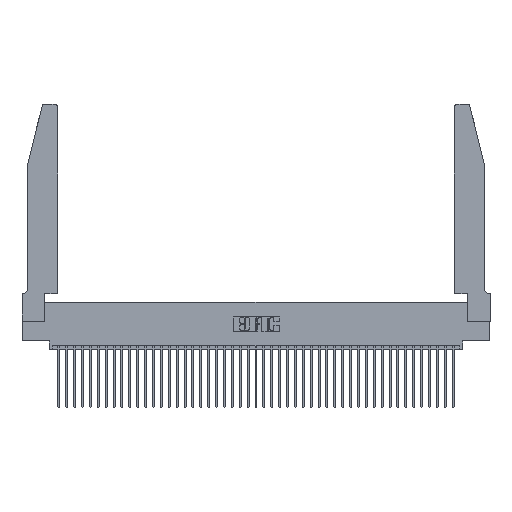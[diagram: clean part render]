
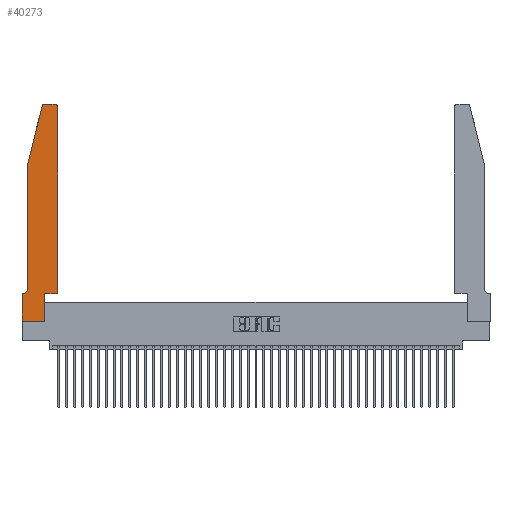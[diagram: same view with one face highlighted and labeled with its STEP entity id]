
A CAD part, top view. The second image highlights one B-rep face of the part: STEP entity #40273.
In plain terms, the highlighted planar face has unit normal (0, 0, 1).
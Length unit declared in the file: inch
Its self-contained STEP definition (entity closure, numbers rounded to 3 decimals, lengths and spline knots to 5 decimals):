
#935 = DIRECTION ( 'NONE',  ( -1., 0., 0. ) ) ;
#1288 = DIRECTION ( 'NONE',  ( 1., 0., 0. ) ) ;
#3307 = DIRECTION ( 'NONE',  ( 0., -1., 0. ) ) ;
#3815 = VERTEX_POINT ( 'NONE', #11834 ) ;
#4508 = CARTESIAN_POINT ( 'NONE',  ( 0.2865, 0., 0.37 ) ) ;
#4598 = EDGE_LOOP ( 'NONE', ( #22814, #32112, #6615, #11169, #37829, #42967, #33319, #41720, #20556, #8556, #37438, #32371 ) ) ;
#5459 = VECTOR ( 'NONE', #7667, 39.37008 ) ;
#5753 = DIRECTION ( 'NONE',  ( 1., 0., 0. ) ) ;
#6615 = ORIENTED_EDGE ( 'NONE', *, *, #26195, .T. ) ;
#6914 = DIRECTION ( 'NONE',  ( 1., 0., 0. ) ) ;
#7610 = CARTESIAN_POINT ( 'NONE',  ( 0.0755, 2., 0.37 ) ) ;
#7634 = CARTESIAN_POINT ( 'NONE',  ( 0., 0., 0.37 ) ) ;
#7667 = DIRECTION ( 'NONE',  ( -1., 0., 0. ) ) ;
#8154 = EDGE_CURVE ( 'NONE', #12439, #22724, #13088, .T. ) ;
#8410 = VERTEX_POINT ( 'NONE', #4508 ) ;
#8518 = CARTESIAN_POINT ( 'NONE',  ( 0.2865, 0.35, 0.37 ) ) ;
#8556 = ORIENTED_EDGE ( 'NONE', *, *, #33210, .T. ) ;
#9580 = CARTESIAN_POINT ( 'NONE',  ( 0.4205, 2.75, 0.37 ) ) ;
#9873 = CARTESIAN_POINT ( 'NONE',  ( 0.25487, 2.72718, 0.37 ) ) ;
#10303 = CARTESIAN_POINT ( 'NONE',  ( 0.2605, 2.75, 0.37 ) ) ;
#10686 = VECTOR ( 'NONE', #33899, 39.37008 ) ;
#11095 = EDGE_CURVE ( 'NONE', #3815, #42620, #15480, .T. ) ;
#11169 = ORIENTED_EDGE ( 'NONE', *, *, #31546, .T. ) ;
#11187 = DIRECTION ( 'NONE',  ( -0.239, -0.971, 0. ) ) ;
#11375 = DIRECTION ( 'NONE',  ( 0., 1., 0. ) ) ;
#11556 = VERTEX_POINT ( 'NONE', #36899 ) ;
#11834 = CARTESIAN_POINT ( 'NONE',  ( 0., 0.35, 0.37 ) ) ;
#12362 = VERTEX_POINT ( 'NONE', #9580 ) ;
#12417 = CARTESIAN_POINT ( 'NONE',  ( 0.4505, 0.35, 0.37 ) ) ;
#12439 = VERTEX_POINT ( 'NONE', #29566 ) ;
#12839 = LINE ( 'NONE', #12417, #37230 ) ;
#13063 = AXIS2_PLACEMENT_3D ( 'NONE', #14311, #21127, #935 ) ;
#13088 = CIRCLE ( 'NONE', #13063, 0.07 ) ;
#13174 = AXIS2_PLACEMENT_3D ( 'NONE', #28355, #38923, #1288 ) ;
#13742 = LINE ( 'NONE', #7610, #37541 ) ;
#14163 = CARTESIAN_POINT ( 'NONE',  ( 0.284, 2.72, 0.37 ) ) ;
#14311 = CARTESIAN_POINT ( 'NONE',  ( 0.0055, 0.42, 0.37 ) ) ;
#14461 = LINE ( 'NONE', #26041, #5459 ) ;
#15480 = LINE ( 'NONE', #23377, #32351 ) ;
#16044 = VERTEX_POINT ( 'NONE', #9873 ) ;
#16285 = DIRECTION ( 'NONE',  ( 0., -1., 0. ) ) ;
#16552 = CARTESIAN_POINT ( 'NONE',  ( 0.0055, 0.35, 0.37 ) ) ;
#16766 = CARTESIAN_POINT ( 'NONE',  ( 0.0755, 2., 0.37 ) ) ;
#17134 = CARTESIAN_POINT ( 'NONE',  ( 0.4205, 2.72, 0.37 ) ) ;
#18446 = VERTEX_POINT ( 'NONE', #36794 ) ;
#18506 = EDGE_CURVE ( 'NONE', #11556, #12362, #42036, .T. ) ;
#18605 = CARTESIAN_POINT ( 'NONE',  ( 0.2865, 0.35, 0.37 ) ) ;
#18828 = VECTOR ( 'NONE', #21265, 39.37008 ) ;
#20556 = ORIENTED_EDGE ( 'NONE', *, *, #22803, .T. ) ;
#21127 = DIRECTION ( 'NONE',  ( 0., 0., -1. ) ) ;
#21265 = DIRECTION ( 'NONE',  ( 0., 1., 0. ) ) ;
#21495 = PLANE ( 'NONE',  #13174 ) ;
#22724 = VERTEX_POINT ( 'NONE', #16552 ) ;
#22786 = VERTEX_POINT ( 'NONE', #30596 ) ;
#22803 = EDGE_CURVE ( 'NONE', #8410, #24852, #27697, .T. ) ;
#22814 = ORIENTED_EDGE ( 'NONE', *, *, #32704, .T. ) ;
#22847 = VERTEX_POINT ( 'NONE', #28722 ) ;
#23377 = CARTESIAN_POINT ( 'NONE',  ( 0., 0., 0.37 ) ) ;
#23465 = LINE ( 'NONE', #7634, #33442 ) ;
#24453 = FACE_OUTER_BOUND ( 'NONE', #4598, .T. ) ;
#24516 = DIRECTION ( 'NONE',  ( 0., 0., 1. ) ) ;
#24852 = VERTEX_POINT ( 'NONE', #8518 ) ;
#25799 = LINE ( 'NONE', #10303, #10686 ) ;
#26041 = CARTESIAN_POINT ( 'NONE',  ( 0.0755, 0.35, 0.37 ) ) ;
#26195 = EDGE_CURVE ( 'NONE', #16044, #18446, #13742, .T. ) ;
#27302 = EDGE_CURVE ( 'NONE', #22786, #11556, #34080, .T. ) ;
#27320 = EDGE_CURVE ( 'NONE', #22847, #16044, #33566, .T. ) ;
#27697 = LINE ( 'NONE', #18605, #43117 ) ;
#28355 = CARTESIAN_POINT ( 'NONE',  ( 0., 0.35, 0.37 ) ) ;
#28458 = CARTESIAN_POINT ( 'NONE',  ( 0., 0., 0.37 ) ) ;
#28722 = CARTESIAN_POINT ( 'NONE',  ( 0.284, 2.75, 0.37 ) ) ;
#29072 = AXIS2_PLACEMENT_3D ( 'NONE', #17134, #33640, #6914 ) ;
#29566 = CARTESIAN_POINT ( 'NONE',  ( 0.0755, 0.42, 0.37 ) ) ;
#30596 = CARTESIAN_POINT ( 'NONE',  ( 0.4505, 0.35, 0.37 ) ) ;
#31546 = EDGE_CURVE ( 'NONE', #18446, #12439, #41779, .T. ) ;
#31552 = CARTESIAN_POINT ( 'NONE',  ( 0.4505, 0.35, 0.37 ) ) ;
#32112 = ORIENTED_EDGE ( 'NONE', *, *, #27320, .T. ) ;
#32351 = VECTOR ( 'NONE', #16285, 39.37008 ) ;
#32371 = ORIENTED_EDGE ( 'NONE', *, *, #18506, .T. ) ;
#32704 = EDGE_CURVE ( 'NONE', #12362, #22847, #25799, .T. ) ;
#32716 = VECTOR ( 'NONE', #3307, 39.37008 ) ;
#32971 = AXIS2_PLACEMENT_3D ( 'NONE', #14163, #24516, #38118 ) ;
#33073 = EDGE_CURVE ( 'NONE', #22724, #3815, #14461, .T. ) ;
#33210 = EDGE_CURVE ( 'NONE', #24852, #22786, #12839, .T. ) ;
#33319 = ORIENTED_EDGE ( 'NONE', *, *, #11095, .T. ) ;
#33442 = VECTOR ( 'NONE', #38101, 39.37008 ) ;
#33566 = CIRCLE ( 'NONE', #32971, 0.03 ) ;
#33640 = DIRECTION ( 'NONE',  ( 0., 0., 1. ) ) ;
#33656 = EDGE_CURVE ( 'NONE', #42620, #8410, #23465, .T. ) ;
#33899 = DIRECTION ( 'NONE',  ( -1., 0., 0. ) ) ;
#34080 = LINE ( 'NONE', #31552, #18828 ) ;
#36794 = CARTESIAN_POINT ( 'NONE',  ( 0.0755, 2., 0.37 ) ) ;
#36899 = CARTESIAN_POINT ( 'NONE',  ( 0.4505, 2.72, 0.37 ) ) ;
#37230 = VECTOR ( 'NONE', #5753, 39.37008 ) ;
#37438 = ORIENTED_EDGE ( 'NONE', *, *, #27302, .T. ) ;
#37541 = VECTOR ( 'NONE', #11187, 39.37008 ) ;
#37829 = ORIENTED_EDGE ( 'NONE', *, *, #8154, .T. ) ;
#38101 = DIRECTION ( 'NONE',  ( 1., 0., 0. ) ) ;
#38118 = DIRECTION ( 'NONE',  ( 1., 0., 0. ) ) ;
#38923 = DIRECTION ( 'NONE',  ( 0., 0., 1. ) ) ;
#40273 = ADVANCED_FACE ( 'NONE', ( #24453 ), #21495, .T. ) ;
#41720 = ORIENTED_EDGE ( 'NONE', *, *, #33656, .T. ) ;
#41779 = LINE ( 'NONE', #16766, #32716 ) ;
#42036 = CIRCLE ( 'NONE', #29072, 0.03 ) ;
#42620 = VERTEX_POINT ( 'NONE', #28458 ) ;
#42967 = ORIENTED_EDGE ( 'NONE', *, *, #33073, .T. ) ;
#43117 = VECTOR ( 'NONE', #11375, 39.37008 ) ;
